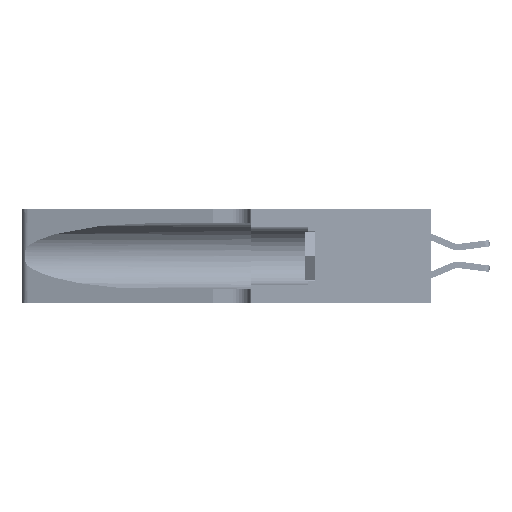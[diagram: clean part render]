
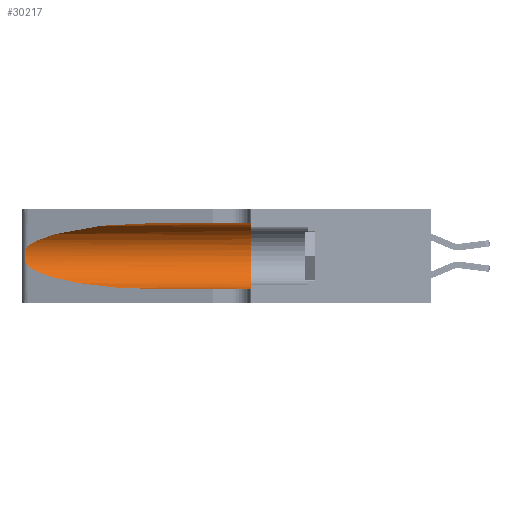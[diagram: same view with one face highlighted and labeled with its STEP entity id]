
A CAD part, left-side view. The second image highlights one B-rep face of the part: STEP entity #30217.
In plain terms, the highlighted cylindrical face has radius 3.308 mm (diameter 6.617 mm), a partial arc.
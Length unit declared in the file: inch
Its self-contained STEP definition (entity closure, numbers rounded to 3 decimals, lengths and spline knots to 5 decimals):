
#1545 = EDGE_CURVE ( 'NONE', #31837, #27598, #38047, .T. ) ;
#1991 = LINE ( 'NONE', #26072, #39833 ) ;
#2279 = CARTESIAN_POINT ( 'NONE',  ( 0.25854, 1.2359, 0.20912 ) ) ;
#4109 = AXIS2_PLACEMENT_3D ( 'NONE', #26334, #4940, #43875 ) ;
#4202 = EDGE_LOOP ( 'NONE', ( #4459, #5288, #5469, #5727, #7901, #8124 ) ) ;
#4459 = ORIENTED_EDGE ( 'NONE', *, *, #5063, .T. ) ;
#4690 = DIRECTION ( 'NONE',  ( 0., -1., 0. ) ) ;
#4940 = DIRECTION ( 'NONE',  ( 0., -1., 0. ) ) ;
#5063 = EDGE_CURVE ( 'NONE', #13557, #31837, #13957, .T. ) ;
#5288 = ORIENTED_EDGE ( 'NONE', *, *, #1545, .T. ) ;
#5469 = ORIENTED_EDGE ( 'NONE', *, *, #26607, .T. ) ;
#5651 = CARTESIAN_POINT ( 'NONE',  ( 0.25487, 1.22718, 0.14631 ) ) ;
#5727 = ORIENTED_EDGE ( 'NONE', *, *, #12712, .T. ) ;
#5905 = CARTESIAN_POINT ( 'NONE',  ( 0.26075, 1.23896, 0.19203 ) ) ;
#6228 = CARTESIAN_POINT ( 'NONE',  ( 0.1305, 0.35, 0.31525 ) ) ;
#6558 = AXIS2_PLACEMENT_3D ( 'NONE', #7975, #32915, #11563 ) ;
#6775 = CARTESIAN_POINT ( 'NONE',  ( 0.1305, 0.72297, 0.31525 ) ) ;
#7453 = VERTEX_POINT ( 'NONE', #41197 ) ;
#7901 = ORIENTED_EDGE ( 'NONE', *, *, #44650, .F. ) ;
#7975 = CARTESIAN_POINT ( 'NONE',  ( 0.1305, 0.35, 0.185 ) ) ;
#8124 = ORIENTED_EDGE ( 'NONE', *, *, #20554, .F. ) ;
#9489 = CARTESIAN_POINT ( 'NONE',  ( 0.26017, 1.23833, 0.17102 ) ) ;
#10567 = CARTESIAN_POINT ( 'NONE',  ( 0.1305, 1.61858, 0.05475 ) ) ;
#11563 = DIRECTION ( 'NONE',  ( 0., 0., 1. ) ) ;
#11681 = LINE ( 'NONE', #10567, #37804 ) ;
#12712 = EDGE_CURVE ( 'NONE', #7453, #18522, #11681, .T. ) ;
#12919 = CARTESIAN_POINT ( 'NONE',  ( 0.25487, 1.22718, 0.22369 ) ) ;
#13074 = CARTESIAN_POINT ( 'NONE',  ( 0.25789, 1.23486, 0.15765 ) ) ;
#13557 = VERTEX_POINT ( 'NONE', #22102 ) ;
#13957 =( BOUNDED_CURVE ( )  B_SPLINE_CURVE ( 3, ( #6775, #28139, #38801, #17600 ),
 .UNSPECIFIED., .F., .F. ) 
 B_SPLINE_CURVE_WITH_KNOTS ( ( 4, 4 ),
 ( 1.5708, 2.84003 ),
 .UNSPECIFIED. ) 
 CURVE ( )  GEOMETRIC_REPRESENTATION_ITEM ( )  RATIONAL_B_SPLINE_CURVE ( ( 1., 0.87, 0.87, 1. ) ) 
 REPRESENTATION_ITEM ( '' )  );
#14014 = FACE_OUTER_BOUND ( 'NONE', #4202, .T. ) ;
#16697 = CARTESIAN_POINT ( 'NONE',  ( 0.25555, 1.22993, 0.14849 ) ) ;
#16839 = CIRCLE ( 'NONE', #6558, 0.13025 ) ;
#17600 = CARTESIAN_POINT ( 'NONE',  ( 0.25487, 1.22718, 0.22369 ) ) ;
#18100 = CARTESIAN_POINT ( 'NONE',  ( 0.18966, 0.96281, 0.05475 ) ) ;
#18522 = VERTEX_POINT ( 'NONE', #22380 ) ;
#18853 = VERTEX_POINT ( 'NONE', #6228 ) ;
#20151 = CARTESIAN_POINT ( 'NONE',  ( 0.25555, 1.22994, 0.2215 ) ) ;
#20554 = EDGE_CURVE ( 'NONE', #13557, #18853, #1991, .T. ) ;
#21081 = CARTESIAN_POINT ( 'NONE',  ( 0.25487, 1.22718, 0.22369 ) ) ;
#22102 = CARTESIAN_POINT ( 'NONE',  ( 0.1305, 0.72297, 0.31525 ) ) ;
#22380 = CARTESIAN_POINT ( 'NONE',  ( 0.1305, 0.35, 0.05475 ) ) ;
#23707 = CARTESIAN_POINT ( 'NONE',  ( 0.25787, 1.23484, 0.2124 ) ) ;
#24791 = DIRECTION ( 'NONE',  ( 0., -1., 0. ) ) ;
#26072 = CARTESIAN_POINT ( 'NONE',  ( 0.1305, 1.61858, 0.31525 ) ) ;
#26334 = CARTESIAN_POINT ( 'NONE',  ( 0.1305, 1.61858, 0.185 ) ) ;
#26607 = EDGE_CURVE ( 'NONE', #27598, #7453, #45730, .T. ) ;
#27288 = CARTESIAN_POINT ( 'NONE',  ( 0.26018, 1.23835, 0.19895 ) ) ;
#27598 = VERTEX_POINT ( 'NONE', #5651 ) ;
#28139 = CARTESIAN_POINT ( 'NONE',  ( 0.18966, 0.96281, 0.31525 ) ) ;
#30217 = ADVANCED_FACE ( 'NONE', ( #14014 ), #31826, .F. ) ;
#30839 = CARTESIAN_POINT ( 'NONE',  ( 0.26075, 1.23896, 0.178 ) ) ;
#31826 = CYLINDRICAL_SURFACE ( 'NONE', #4109, 0.13025 ) ;
#31837 = VERTEX_POINT ( 'NONE', #21081 ) ;
#32206 = CARTESIAN_POINT ( 'NONE',  ( 0.25487, 1.22718, 0.14631 ) ) ;
#32915 = DIRECTION ( 'NONE',  ( 0., 1., 0. ) ) ;
#34387 = CARTESIAN_POINT ( 'NONE',  ( 0.25856, 1.23593, 0.16098 ) ) ;
#35743 = CARTESIAN_POINT ( 'NONE',  ( 0.2373, 1.15595, 0.08982 ) ) ;
#37804 = VECTOR ( 'NONE', #24791, 39.37008 ) ;
#37922 = CARTESIAN_POINT ( 'NONE',  ( 0.25639, 1.23186, 0.15144 ) ) ;
#38047 = B_SPLINE_CURVE_WITH_KNOTS ( 'NONE', 3,
 ( #12919, #20151, #44810, #23707, #2279, #27288, #5905, #30839, #9489, #34387, #13074, #37922, #16697, #41423 ),
 .UNSPECIFIED., .F., .F.,
 ( 4, 2, 2, 2, 2, 2, 4 ),
 ( 0., 0.00027, 0.00053, 0.00107, 0.0016, 0.00187, 0.00214 ),
 .UNSPECIFIED. ) ;
#38801 = CARTESIAN_POINT ( 'NONE',  ( 0.2373, 1.15595, 0.28018 ) ) ;
#39833 = VECTOR ( 'NONE', #4690, 39.37008 ) ;
#41197 = CARTESIAN_POINT ( 'NONE',  ( 0.1305, 0.72297, 0.05475 ) ) ;
#41423 = CARTESIAN_POINT ( 'NONE',  ( 0.25487, 1.22718, 0.14631 ) ) ;
#42792 = CARTESIAN_POINT ( 'NONE',  ( 0.1305, 0.72297, 0.05475 ) ) ;
#43875 = DIRECTION ( 'NONE',  ( 0., 0., -1. ) ) ;
#44650 = EDGE_CURVE ( 'NONE', #18853, #18522, #16839, .T. ) ;
#44810 = CARTESIAN_POINT ( 'NONE',  ( 0.25639, 1.23184, 0.21858 ) ) ;
#45730 =( BOUNDED_CURVE ( )  B_SPLINE_CURVE ( 3, ( #32206, #35743, #18100, #42792 ),
 .UNSPECIFIED., .F., .T. ) 
 B_SPLINE_CURVE_WITH_KNOTS ( ( 4, 4 ),
 ( 3.44316, 4.71239 ),
 .UNSPECIFIED. ) 
 CURVE ( )  GEOMETRIC_REPRESENTATION_ITEM ( )  RATIONAL_B_SPLINE_CURVE ( ( 1., 0.87, 0.87, 1. ) ) 
 REPRESENTATION_ITEM ( '' )  );
